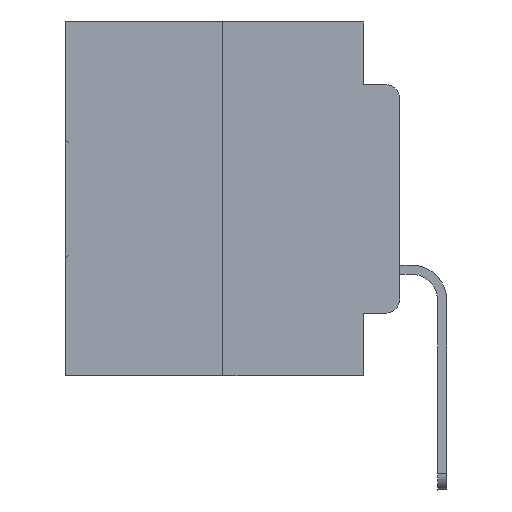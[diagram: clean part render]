
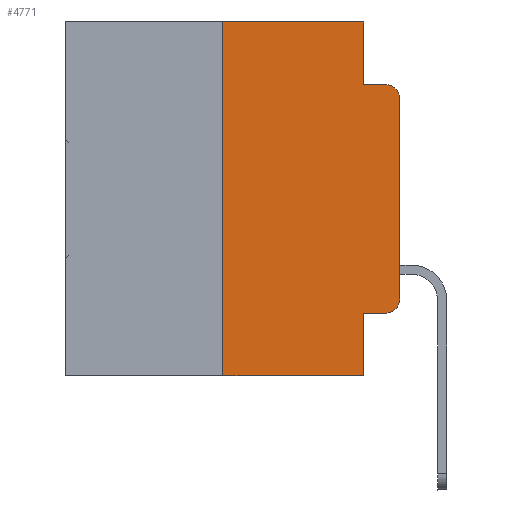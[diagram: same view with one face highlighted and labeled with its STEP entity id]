
A CAD part, left-side view. The second image highlights one B-rep face of the part: STEP entity #4771.
In plain terms, the highlighted planar face has unit normal (-1, 0, 0).
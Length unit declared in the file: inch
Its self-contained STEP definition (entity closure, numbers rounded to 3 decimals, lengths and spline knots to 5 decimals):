
#105 = DIRECTION ( 'NONE',  ( 0., -1., 0. ) ) ;
#343 = CARTESIAN_POINT ( 'NONE',  ( 0., 0.051, -0.0885 ) ) ;
#1049 = CARTESIAN_POINT ( 'NONE',  ( 0., 0., -0.1085 ) ) ;
#1116 = DIRECTION ( 'NONE',  ( -1., 0., 0. ) ) ;
#1143 = CARTESIAN_POINT ( 'NONE',  ( 0., 0.02, -0.0885 ) ) ;
#1803 = EDGE_CURVE ( 'NONE', #11942, #6966, #2829, .T. ) ;
#1835 = CARTESIAN_POINT ( 'NONE',  ( 0., 0.25, 0. ) ) ;
#1916 = DIRECTION ( 'NONE',  ( 0., -1., 0. ) ) ;
#2211 = DIRECTION ( 'NONE',  ( 0., 0., -1. ) ) ;
#2392 = CARTESIAN_POINT ( 'NONE',  ( 0., 0.02, -0.4115 ) ) ;
#2829 = LINE ( 'NONE', #21438, #26309 ) ;
#2875 = CIRCLE ( 'NONE', #26645, 0.02 ) ;
#2951 = VECTOR ( 'NONE', #22872, 39.37008 ) ;
#3276 = DIRECTION ( 'NONE',  ( 0., 0., -1. ) ) ;
#3785 = PLANE ( 'NONE',  #29156 ) ;
#3818 = EDGE_CURVE ( 'NONE', #25462, #15028, #24800, .T. ) ;
#3979 = LINE ( 'NONE', #6160, #2951 ) ;
#4771 = ADVANCED_FACE ( 'NONE', ( #15894 ), #3785, .F. ) ;
#5330 = CARTESIAN_POINT ( 'NONE',  ( 0., 0.051, 0. ) ) ;
#6160 = CARTESIAN_POINT ( 'NONE',  ( 0., 0., 0. ) ) ;
#6229 = VERTEX_POINT ( 'NONE', #1049 ) ;
#6888 = EDGE_CURVE ( 'NONE', #19038, #11942, #28401, .T. ) ;
#6945 = DIRECTION ( 'NONE',  ( 0., -1., 0. ) ) ;
#6966 = VERTEX_POINT ( 'NONE', #343 ) ;
#7049 = CARTESIAN_POINT ( 'NONE',  ( 0., 0.473, 0. ) ) ;
#7748 = EDGE_CURVE ( 'NONE', #25462, #19038, #28333, .T. ) ;
#8235 = ORIENTED_EDGE ( 'NONE', *, *, #21481, .T. ) ;
#8255 = VECTOR ( 'NONE', #105, 39.37008 ) ;
#8350 = EDGE_CURVE ( 'NONE', #21848, #15028, #12609, .T. ) ;
#9197 = CARTESIAN_POINT ( 'NONE',  ( 0., 0.02, -0.1085 ) ) ;
#9522 = DIRECTION ( 'NONE',  ( -1., 0., 0. ) ) ;
#9889 = CARTESIAN_POINT ( 'NONE',  ( 0., 0.051, -0.4115 ) ) ;
#11023 = ORIENTED_EDGE ( 'NONE', *, *, #14868, .T. ) ;
#11096 = DIRECTION ( 'NONE',  ( 1., 0., 0. ) ) ;
#11942 = VERTEX_POINT ( 'NONE', #27610 ) ;
#11958 = ORIENTED_EDGE ( 'NONE', *, *, #1803, .F. ) ;
#12045 = CARTESIAN_POINT ( 'NONE',  ( 0., 0.051, -0.0885 ) ) ;
#12609 = LINE ( 'NONE', #5330, #29775 ) ;
#13221 = ORIENTED_EDGE ( 'NONE', *, *, #3818, .T. ) ;
#13251 = CARTESIAN_POINT ( 'NONE',  ( 0., 0.473, 0. ) ) ;
#13782 = DIRECTION ( 'NONE',  ( 0., 0., 1. ) ) ;
#14784 = DIRECTION ( 'NONE',  ( 0., 0., -1. ) ) ;
#14868 = EDGE_CURVE ( 'NONE', #19949, #20829, #24038, .T. ) ;
#15028 = VERTEX_POINT ( 'NONE', #17045 ) ;
#15836 = CARTESIAN_POINT ( 'NONE',  ( 0., 0.051, -0.4115 ) ) ;
#15894 = FACE_OUTER_BOUND ( 'NONE', #29220, .T. ) ;
#16020 = ORIENTED_EDGE ( 'NONE', *, *, #28531, .T. ) ;
#16399 = VECTOR ( 'NONE', #13782, 39.37008 ) ;
#16585 = ORIENTED_EDGE ( 'NONE', *, *, #7748, .F. ) ;
#16733 = CARTESIAN_POINT ( 'NONE',  ( 0., 0.25, 0. ) ) ;
#17045 = CARTESIAN_POINT ( 'NONE',  ( 0., 0.051, -0.5 ) ) ;
#19038 = VERTEX_POINT ( 'NONE', #16733 ) ;
#19346 = CARTESIAN_POINT ( 'NONE',  ( 0., 0., -0.3915 ) ) ;
#19949 = VERTEX_POINT ( 'NONE', #2392 ) ;
#20155 = CARTESIAN_POINT ( 'NONE',  ( 0., 0.473, -0.5 ) ) ;
#20286 = EDGE_CURVE ( 'NONE', #6229, #27696, #2875, .T. ) ;
#20538 = DIRECTION ( 'NONE',  ( 0., 0., -1. ) ) ;
#20829 = VERTEX_POINT ( 'NONE', #19346 ) ;
#21438 = CARTESIAN_POINT ( 'NONE',  ( 0., 0.051, 0. ) ) ;
#21481 = EDGE_CURVE ( 'NONE', #20829, #6229, #3979, .T. ) ;
#21630 = LINE ( 'NONE', #9889, #8255 ) ;
#21848 = VERTEX_POINT ( 'NONE', #15836 ) ;
#22351 = CARTESIAN_POINT ( 'NONE',  ( 0., 0.02, -0.3915 ) ) ;
#22422 = ORIENTED_EDGE ( 'NONE', *, *, #20286, .T. ) ;
#22822 = ORIENTED_EDGE ( 'NONE', *, *, #6888, .F. ) ;
#22872 = DIRECTION ( 'NONE',  ( 0., 0., 1. ) ) ;
#23699 = ORIENTED_EDGE ( 'NONE', *, *, #8350, .F. ) ;
#24038 = CIRCLE ( 'NONE', #29496, 0.02 ) ;
#24800 = LINE ( 'NONE', #20155, #29948 ) ;
#25462 = VERTEX_POINT ( 'NONE', #28808 ) ;
#25924 = EDGE_CURVE ( 'NONE', #6966, #27696, #26291, .T. ) ;
#26291 = LINE ( 'NONE', #12045, #27698 ) ;
#26309 = VECTOR ( 'NONE', #28264, 39.37008 ) ;
#26645 = AXIS2_PLACEMENT_3D ( 'NONE', #9197, #9522, #2211 ) ;
#26679 = DIRECTION ( 'NONE',  ( 0., -1., 0. ) ) ;
#26755 = VECTOR ( 'NONE', #1916, 39.37008 ) ;
#27610 = CARTESIAN_POINT ( 'NONE',  ( 0., 0.051, 0. ) ) ;
#27624 = ORIENTED_EDGE ( 'NONE', *, *, #25924, .F. ) ;
#27696 = VERTEX_POINT ( 'NONE', #1143 ) ;
#27698 = VECTOR ( 'NONE', #6945, 39.37008 ) ;
#28264 = DIRECTION ( 'NONE',  ( 0., 0., -1. ) ) ;
#28333 = LINE ( 'NONE', #1835, #16399 ) ;
#28401 = LINE ( 'NONE', #7049, #26755 ) ;
#28531 = EDGE_CURVE ( 'NONE', #21848, #19949, #21630, .T. ) ;
#28808 = CARTESIAN_POINT ( 'NONE',  ( 0., 0.25, -0.5 ) ) ;
#29156 = AXIS2_PLACEMENT_3D ( 'NONE', #13251, #11096, #20538 ) ;
#29220 = EDGE_LOOP ( 'NONE', ( #8235, #22422, #27624, #11958, #22822, #16585, #13221, #23699, #16020, #11023 ) ) ;
#29496 = AXIS2_PLACEMENT_3D ( 'NONE', #22351, #1116, #3276 ) ;
#29775 = VECTOR ( 'NONE', #14784, 39.37008 ) ;
#29948 = VECTOR ( 'NONE', #26679, 39.37008 ) ;
